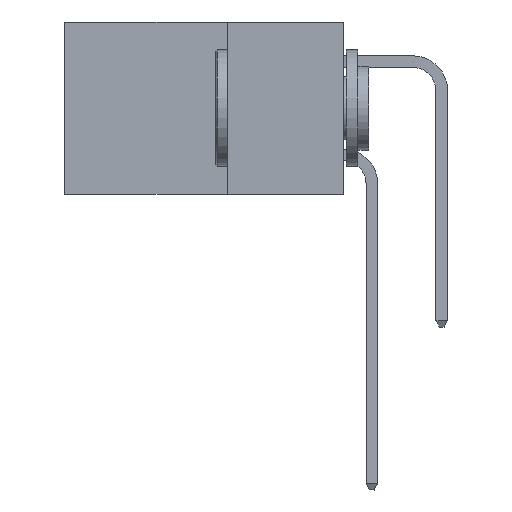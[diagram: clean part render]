
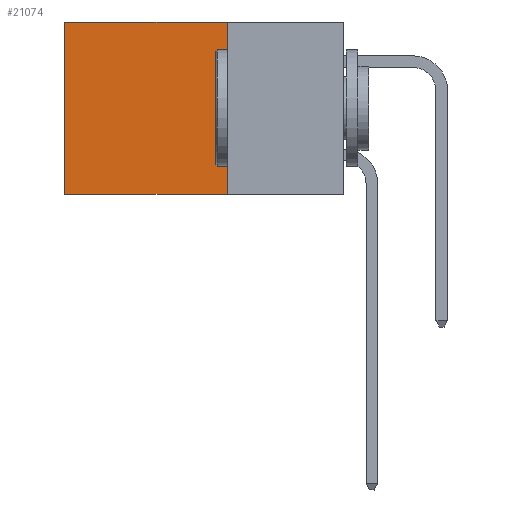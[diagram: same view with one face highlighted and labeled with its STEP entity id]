
A CAD part, left-side view. The second image highlights one B-rep face of the part: STEP entity #21074.
In plain terms, the highlighted planar face has unit normal (-1, 0, 0).
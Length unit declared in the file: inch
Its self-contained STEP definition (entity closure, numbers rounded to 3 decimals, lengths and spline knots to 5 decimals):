
#598 = ORIENTED_EDGE ( 'NONE', *, *, #12220, .T. ) ;
#989 = CARTESIAN_POINT ( 'NONE',  ( 0.298, 0.25, 0. ) ) ;
#1074 = DIRECTION ( 'NONE',  ( 0., 0., -1. ) ) ;
#1131 = CARTESIAN_POINT ( 'NONE',  ( 0.298, 0.25, 0. ) ) ;
#2923 = CARTESIAN_POINT ( 'NONE',  ( 0.298, 0.6, 0. ) ) ;
#4505 = VERTEX_POINT ( 'NONE', #20168 ) ;
#5815 = ORIENTED_EDGE ( 'NONE', *, *, #9430, .F. ) ;
#5990 = PLANE ( 'NONE',  #10635 ) ;
#6157 = CARTESIAN_POINT ( 'NONE',  ( 0.298, 0.6, 0. ) ) ;
#6473 = EDGE_CURVE ( 'NONE', #9852, #16444, #13286, .T. ) ;
#6746 = VECTOR ( 'NONE', #15851, 39.37008 ) ;
#6981 = VECTOR ( 'NONE', #10645, 39.37008 ) ;
#7282 = LINE ( 'NONE', #15337, #6746 ) ;
#7929 = VERTEX_POINT ( 'NONE', #6157 ) ;
#9312 = FACE_OUTER_BOUND ( 'NONE', #11692, .T. ) ;
#9430 = EDGE_CURVE ( 'NONE', #16444, #4505, #7282, .T. ) ;
#9852 = VERTEX_POINT ( 'NONE', #1131 ) ;
#10635 = AXIS2_PLACEMENT_3D ( 'NONE', #16069, #11124, #1074 ) ;
#10645 = DIRECTION ( 'NONE',  ( 0., 1., 0. ) ) ;
#11124 = DIRECTION ( 'NONE',  ( 1., 0., 0. ) ) ;
#11494 = LINE ( 'NONE', #12246, #6981 ) ;
#11506 = ORIENTED_EDGE ( 'NONE', *, *, #21146, .T. ) ;
#11692 = EDGE_LOOP ( 'NONE', ( #11506, #5815, #13439, #598 ) ) ;
#12220 = EDGE_CURVE ( 'NONE', #9852, #7929, #11494, .T. ) ;
#12246 = CARTESIAN_POINT ( 'NONE',  ( 0.298, 0.25, 0. ) ) ;
#13286 = LINE ( 'NONE', #989, #17125 ) ;
#13439 = ORIENTED_EDGE ( 'NONE', *, *, #6473, .F. ) ;
#14703 = DIRECTION ( 'NONE',  ( 0., 0., -1. ) ) ;
#15337 = CARTESIAN_POINT ( 'NONE',  ( 0.298, 0.25, -0.37 ) ) ;
#15851 = DIRECTION ( 'NONE',  ( 0., 1., 0. ) ) ;
#16069 = CARTESIAN_POINT ( 'NONE',  ( 0.298, 0.25, 0. ) ) ;
#16085 = LINE ( 'NONE', #2923, #20372 ) ;
#16444 = VERTEX_POINT ( 'NONE', #16654 ) ;
#16654 = CARTESIAN_POINT ( 'NONE',  ( 0.298, 0.25, -0.37 ) ) ;
#17125 = VECTOR ( 'NONE', #21073, 39.37008 ) ;
#20168 = CARTESIAN_POINT ( 'NONE',  ( 0.298, 0.6, -0.37 ) ) ;
#20372 = VECTOR ( 'NONE', #14703, 39.37008 ) ;
#21073 = DIRECTION ( 'NONE',  ( 0., 0., -1. ) ) ;
#21074 = ADVANCED_FACE ( 'NONE', ( #9312 ), #5990, .F. ) ;
#21146 = EDGE_CURVE ( 'NONE', #7929, #4505, #16085, .T. ) ;
